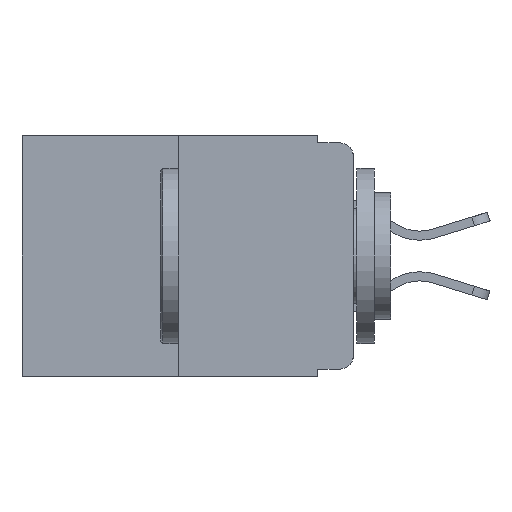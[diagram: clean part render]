
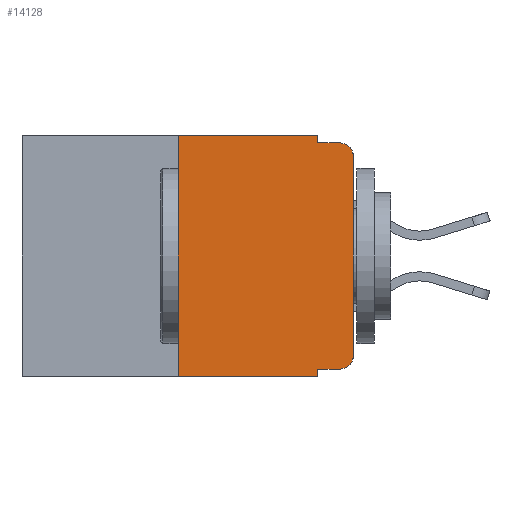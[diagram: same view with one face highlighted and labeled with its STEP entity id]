
A CAD part, left-side view. The second image highlights one B-rep face of the part: STEP entity #14128.
In plain terms, the highlighted planar face has unit normal (-1, 0, 0).
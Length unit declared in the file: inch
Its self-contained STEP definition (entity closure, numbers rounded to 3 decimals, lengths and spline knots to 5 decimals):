
#59 = LINE ( 'NONE', #19493, #17836 ) ;
#281 = LINE ( 'NONE', #11969, #19141 ) ;
#358 = EDGE_CURVE ( 'NONE', #16870, #868, #8005, .T. ) ;
#475 = CARTESIAN_POINT ( 'NONE',  ( 0., 0., -0.313 ) ) ;
#813 = CARTESIAN_POINT ( 'NONE',  ( 0., 0.473, 0. ) ) ;
#868 = VERTEX_POINT ( 'NONE', #19244 ) ;
#942 = DIRECTION ( 'NONE',  ( 0., 0., -1. ) ) ;
#1131 = VECTOR ( 'NONE', #10373, 39.37008 ) ;
#1610 = AXIS2_PLACEMENT_3D ( 'NONE', #13092, #7763, #20064 ) ;
#1655 = CARTESIAN_POINT ( 'NONE',  ( 0., 0.051, -0.01 ) ) ;
#2169 = CARTESIAN_POINT ( 'NONE',  ( 0., 0.051, 0. ) ) ;
#2259 = CARTESIAN_POINT ( 'NONE',  ( 0., 0.02, -0.333 ) ) ;
#2325 = CARTESIAN_POINT ( 'NONE',  ( 0., 0.25, 0. ) ) ;
#2331 = VERTEX_POINT ( 'NONE', #19723 ) ;
#2905 = EDGE_CURVE ( 'NONE', #16870, #7565, #14278, .T. ) ;
#3092 = DIRECTION ( 'NONE',  ( -1., 0., 0. ) ) ;
#3150 = EDGE_LOOP ( 'NONE', ( #8580, #18790, #19867, #14687, #12536, #19099, #21220, #6445, #9015, #11927 ) ) ;
#3153 = VERTEX_POINT ( 'NONE', #475 ) ;
#3306 = VECTOR ( 'NONE', #6066, 39.37008 ) ;
#3873 = FACE_OUTER_BOUND ( 'NONE', #3150, .T. ) ;
#4676 = DIRECTION ( 'NONE',  ( 0., 0., 1. ) ) ;
#6066 = DIRECTION ( 'NONE',  ( 0., 0., -1. ) ) ;
#6445 = ORIENTED_EDGE ( 'NONE', *, *, #14201, .F. ) ;
#7565 = VERTEX_POINT ( 'NONE', #2325 ) ;
#7763 = DIRECTION ( 'NONE',  ( 1., 0., 0. ) ) ;
#8005 = LINE ( 'NONE', #9416, #16848 ) ;
#8022 = VECTOR ( 'NONE', #4676, 39.37008 ) ;
#8195 = VERTEX_POINT ( 'NONE', #16646 ) ;
#8409 = EDGE_CURVE ( 'NONE', #13421, #8195, #281, .T. ) ;
#8580 = ORIENTED_EDGE ( 'NONE', *, *, #22431, .T. ) ;
#9015 = ORIENTED_EDGE ( 'NONE', *, *, #13467, .T. ) ;
#9380 = CIRCLE ( 'NONE', #18187, 0.02 ) ;
#9416 = CARTESIAN_POINT ( 'NONE',  ( 0., 0.473, -0.343 ) ) ;
#10112 = VERTEX_POINT ( 'NONE', #2259 ) ;
#10116 = CARTESIAN_POINT ( 'NONE',  ( 0., 0.25, 0. ) ) ;
#10245 = EDGE_CURVE ( 'NONE', #7565, #15955, #22494, .T. ) ;
#10373 = DIRECTION ( 'NONE',  ( 0., 0., 1. ) ) ;
#11672 = DIRECTION ( 'NONE',  ( -1., 0., 0. ) ) ;
#11927 = ORIENTED_EDGE ( 'NONE', *, *, #17399, .T. ) ;
#11969 = CARTESIAN_POINT ( 'NONE',  ( 0., 0.051, -0.01 ) ) ;
#12064 = VECTOR ( 'NONE', #19356, 39.37008 ) ;
#12536 = ORIENTED_EDGE ( 'NONE', *, *, #10245, .F. ) ;
#12773 = EDGE_CURVE ( 'NONE', #2331, #8195, #22660, .T. ) ;
#13092 = CARTESIAN_POINT ( 'NONE',  ( 0., 0.473, 0. ) ) ;
#13421 = VERTEX_POINT ( 'NONE', #1655 ) ;
#13467 = EDGE_CURVE ( 'NONE', #14809, #10112, #59, .T. ) ;
#13871 = CARTESIAN_POINT ( 'NONE',  ( 0., 0.02, -0.313 ) ) ;
#14128 = ADVANCED_FACE ( 'NONE', ( #3873 ), #16565, .F. ) ;
#14201 = EDGE_CURVE ( 'NONE', #14809, #868, #16424, .T. ) ;
#14253 = DIRECTION ( 'NONE',  ( 0., -1., 0. ) ) ;
#14278 = LINE ( 'NONE', #10116, #1131 ) ;
#14687 = ORIENTED_EDGE ( 'NONE', *, *, #19019, .F. ) ;
#14809 = VERTEX_POINT ( 'NONE', #18454 ) ;
#15367 = CARTESIAN_POINT ( 'NONE',  ( 0., 0., 0. ) ) ;
#15601 = DIRECTION ( 'NONE',  ( 0., 0., -1. ) ) ;
#15955 = VERTEX_POINT ( 'NONE', #2169 ) ;
#16424 = LINE ( 'NONE', #18479, #3306 ) ;
#16565 = PLANE ( 'NONE',  #1610 ) ;
#16610 = DIRECTION ( 'NONE',  ( 0., -1., 0. ) ) ;
#16646 = CARTESIAN_POINT ( 'NONE',  ( 0., 0.02, -0.01 ) ) ;
#16826 = DIRECTION ( 'NONE',  ( 0., -1., 0. ) ) ;
#16848 = VECTOR ( 'NONE', #16610, 39.37008 ) ;
#16870 = VERTEX_POINT ( 'NONE', #21053 ) ;
#17399 = EDGE_CURVE ( 'NONE', #10112, #3153, #9380, .T. ) ;
#17620 = CARTESIAN_POINT ( 'NONE',  ( 0., 0.051, 0. ) ) ;
#17836 = VECTOR ( 'NONE', #14253, 39.37008 ) ;
#18187 = AXIS2_PLACEMENT_3D ( 'NONE', #13871, #3092, #15601 ) ;
#18454 = CARTESIAN_POINT ( 'NONE',  ( 0., 0.051, -0.333 ) ) ;
#18479 = CARTESIAN_POINT ( 'NONE',  ( 0., 0.051, 0. ) ) ;
#18790 = ORIENTED_EDGE ( 'NONE', *, *, #12773, .T. ) ;
#19019 = EDGE_CURVE ( 'NONE', #15955, #13421, #20763, .T. ) ;
#19099 = ORIENTED_EDGE ( 'NONE', *, *, #2905, .F. ) ;
#19141 = VECTOR ( 'NONE', #22319, 39.37008 ) ;
#19244 = CARTESIAN_POINT ( 'NONE',  ( 0., 0.051, -0.343 ) ) ;
#19356 = DIRECTION ( 'NONE',  ( 0., 0., -1. ) ) ;
#19493 = CARTESIAN_POINT ( 'NONE',  ( 0., 0.051, -0.333 ) ) ;
#19723 = CARTESIAN_POINT ( 'NONE',  ( 0., 0., -0.03 ) ) ;
#19867 = ORIENTED_EDGE ( 'NONE', *, *, #8409, .F. ) ;
#20064 = DIRECTION ( 'NONE',  ( 0., 0., -1. ) ) ;
#20763 = LINE ( 'NONE', #17620, #12064 ) ;
#20830 = AXIS2_PLACEMENT_3D ( 'NONE', #22024, #11672, #942 ) ;
#20894 = LINE ( 'NONE', #15367, #8022 ) ;
#21053 = CARTESIAN_POINT ( 'NONE',  ( 0., 0.25, -0.343 ) ) ;
#21220 = ORIENTED_EDGE ( 'NONE', *, *, #358, .T. ) ;
#21952 = VECTOR ( 'NONE', #16826, 39.37008 ) ;
#22024 = CARTESIAN_POINT ( 'NONE',  ( 0., 0.02, -0.03 ) ) ;
#22319 = DIRECTION ( 'NONE',  ( 0., -1., 0. ) ) ;
#22431 = EDGE_CURVE ( 'NONE', #3153, #2331, #20894, .T. ) ;
#22494 = LINE ( 'NONE', #813, #21952 ) ;
#22660 = CIRCLE ( 'NONE', #20830, 0.02 ) ;
